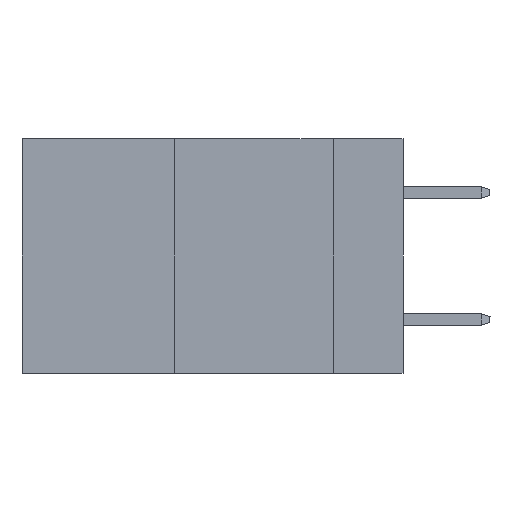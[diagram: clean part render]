
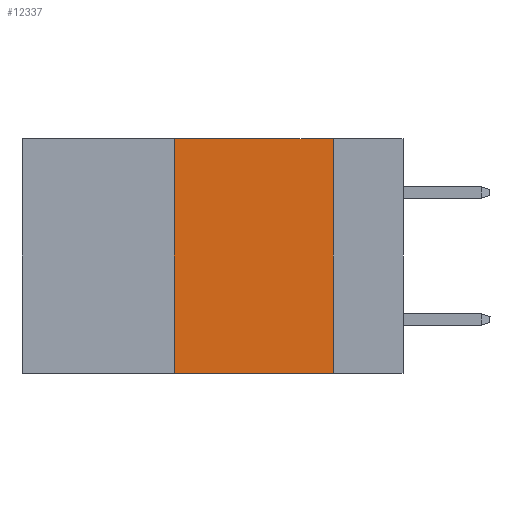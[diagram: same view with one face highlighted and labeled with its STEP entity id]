
A CAD part, left-side view. The second image highlights one B-rep face of the part: STEP entity #12337.
In plain terms, the highlighted planar face has unit normal (-1, 0, 0).
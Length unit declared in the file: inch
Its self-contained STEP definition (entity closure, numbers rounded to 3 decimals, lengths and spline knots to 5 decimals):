
#219 = AXIS2_PLACEMENT_3D ( 'NONE', #5163, #4917, #6792 ) ;
#624 = LINE ( 'NONE', #6400, #10899 ) ;
#992 = LINE ( 'NONE', #10874, #17670 ) ;
#1356 = DIRECTION ( 'NONE',  ( 0., -1., 0. ) ) ;
#2695 = VERTEX_POINT ( 'NONE', #7660 ) ;
#2915 = EDGE_CURVE ( 'NONE', #10674, #14002, #992, .T. ) ;
#3304 = EDGE_LOOP ( 'NONE', ( #21585, #19891, #20531, #13158 ) ) ;
#4917 = DIRECTION ( 'NONE',  ( 1., 0., 0. ) ) ;
#5163 = CARTESIAN_POINT ( 'NONE',  ( 0., 0.6, 0. ) ) ;
#6400 = CARTESIAN_POINT ( 'NONE',  ( 0., 0.11, 0. ) ) ;
#6469 = LINE ( 'NONE', #15647, #24604 ) ;
#6792 = DIRECTION ( 'NONE',  ( 0., 0., -1. ) ) ;
#7660 = CARTESIAN_POINT ( 'NONE',  ( 0., 0.11, -0.37 ) ) ;
#10674 = VERTEX_POINT ( 'NONE', #14738 ) ;
#10874 = CARTESIAN_POINT ( 'NONE',  ( 0., 0.6, 0. ) ) ;
#10899 = VECTOR ( 'NONE', #11792, 39.37008 ) ;
#11792 = DIRECTION ( 'NONE',  ( 0., 0., -1. ) ) ;
#11968 = DIRECTION ( 'NONE',  ( 0., -1., 0. ) ) ;
#12337 = ADVANCED_FACE ( 'NONE', ( #12695 ), #16461, .F. ) ;
#12695 = FACE_OUTER_BOUND ( 'NONE', #3304, .T. ) ;
#12773 = CARTESIAN_POINT ( 'NONE',  ( 0., 0.11, 0. ) ) ;
#12924 = EDGE_CURVE ( 'NONE', #14318, #10674, #6469, .T. ) ;
#13158 = ORIENTED_EDGE ( 'NONE', *, *, #21505, .T. ) ;
#13489 = CARTESIAN_POINT ( 'NONE',  ( 0., 0.6, -0.37 ) ) ;
#14002 = VERTEX_POINT ( 'NONE', #12773 ) ;
#14318 = VERTEX_POINT ( 'NONE', #16130 ) ;
#14738 = CARTESIAN_POINT ( 'NONE',  ( 0., 0.36, 0. ) ) ;
#15647 = CARTESIAN_POINT ( 'NONE',  ( 0., 0.36, 0. ) ) ;
#16130 = CARTESIAN_POINT ( 'NONE',  ( 0., 0.36, -0.37 ) ) ;
#16461 = PLANE ( 'NONE',  #219 ) ;
#17670 = VECTOR ( 'NONE', #1356, 39.37008 ) ;
#17752 = VECTOR ( 'NONE', #11968, 39.37008 ) ;
#19112 = LINE ( 'NONE', #13489, #17752 ) ;
#19891 = ORIENTED_EDGE ( 'NONE', *, *, #2915, .F. ) ;
#20531 = ORIENTED_EDGE ( 'NONE', *, *, #12924, .F. ) ;
#21315 = EDGE_CURVE ( 'NONE', #14002, #2695, #624, .T. ) ;
#21505 = EDGE_CURVE ( 'NONE', #14318, #2695, #19112, .T. ) ;
#21585 = ORIENTED_EDGE ( 'NONE', *, *, #21315, .F. ) ;
#23210 = DIRECTION ( 'NONE',  ( 0., 0., 1. ) ) ;
#24604 = VECTOR ( 'NONE', #23210, 39.37008 ) ;
